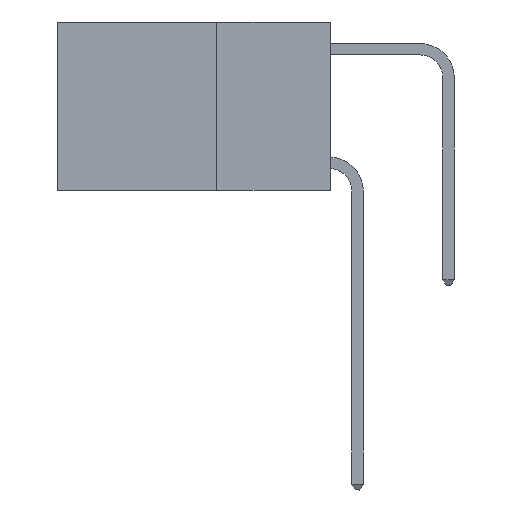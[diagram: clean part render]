
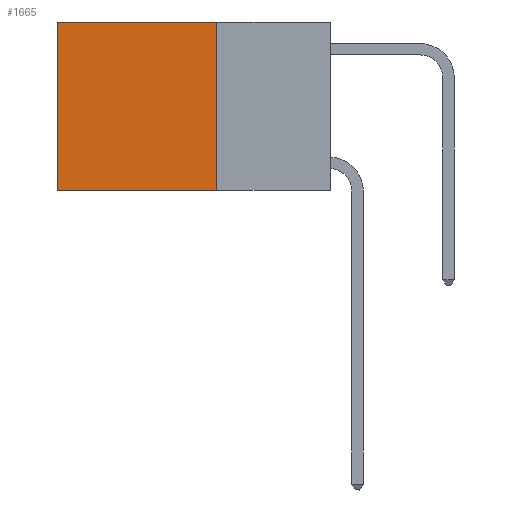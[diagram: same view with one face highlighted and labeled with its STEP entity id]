
A CAD part, left-side view. The second image highlights one B-rep face of the part: STEP entity #1665.
In plain terms, the highlighted planar face has unit normal (-1, 0, 0).
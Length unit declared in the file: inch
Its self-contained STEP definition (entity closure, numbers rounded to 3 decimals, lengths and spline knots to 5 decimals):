
#321 = CARTESIAN_POINT ( 'NONE',  ( 0.2625, 0.25, 0. ) ) ;
#645 = VERTEX_POINT ( 'NONE', #1458 ) ;
#806 = CARTESIAN_POINT ( 'NONE',  ( 0.2625, 0.25, 0. ) ) ;
#1071 = EDGE_CURVE ( 'NONE', #1462, #13157, #5815, .T. ) ;
#1458 = CARTESIAN_POINT ( 'NONE',  ( 0.2625, 0.25, -0.37 ) ) ;
#1462 = VERTEX_POINT ( 'NONE', #11399 ) ;
#1665 = ADVANCED_FACE ( 'NONE', ( #7680 ), #9579, .F. ) ;
#1980 = ORIENTED_EDGE ( 'NONE', *, *, #11956, .F. ) ;
#2825 = VECTOR ( 'NONE', #4287, 39.37008 ) ;
#3129 = ORIENTED_EDGE ( 'NONE', *, *, #9845, .F. ) ;
#3473 = CARTESIAN_POINT ( 'NONE',  ( 0.2625, 0.25, -0.37 ) ) ;
#3650 = AXIS2_PLACEMENT_3D ( 'NONE', #9532, #11773, #5239 ) ;
#3953 = VERTEX_POINT ( 'NONE', #7006 ) ;
#4017 = VECTOR ( 'NONE', #12225, 39.37008 ) ;
#4287 = DIRECTION ( 'NONE',  ( 0., 1., 0. ) ) ;
#4433 = LINE ( 'NONE', #5861, #7014 ) ;
#4465 = CARTESIAN_POINT ( 'NONE',  ( 0.2625, 0.6, 0. ) ) ;
#5239 = DIRECTION ( 'NONE',  ( 0., 0., -1. ) ) ;
#5815 = LINE ( 'NONE', #806, #2825 ) ;
#5861 = CARTESIAN_POINT ( 'NONE',  ( 0.2625, 0.6, 0. ) ) ;
#6144 = LINE ( 'NONE', #321, #14117 ) ;
#7006 = CARTESIAN_POINT ( 'NONE',  ( 0.2625, 0.6, -0.37 ) ) ;
#7014 = VECTOR ( 'NONE', #12363, 39.37008 ) ;
#7680 = FACE_OUTER_BOUND ( 'NONE', #12498, .T. ) ;
#9129 = EDGE_CURVE ( 'NONE', #13157, #3953, #4433, .T. ) ;
#9277 = DIRECTION ( 'NONE',  ( 0., 0., -1. ) ) ;
#9532 = CARTESIAN_POINT ( 'NONE',  ( 0.2625, 0.25, 0. ) ) ;
#9579 = PLANE ( 'NONE',  #3650 ) ;
#9845 = EDGE_CURVE ( 'NONE', #1462, #645, #6144, .T. ) ;
#10166 = LINE ( 'NONE', #3473, #4017 ) ;
#10486 = ORIENTED_EDGE ( 'NONE', *, *, #9129, .T. ) ;
#11399 = CARTESIAN_POINT ( 'NONE',  ( 0.2625, 0.25, 0. ) ) ;
#11773 = DIRECTION ( 'NONE',  ( 1., 0., 0. ) ) ;
#11956 = EDGE_CURVE ( 'NONE', #645, #3953, #10166, .T. ) ;
#12225 = DIRECTION ( 'NONE',  ( 0., 1., 0. ) ) ;
#12363 = DIRECTION ( 'NONE',  ( 0., 0., -1. ) ) ;
#12498 = EDGE_LOOP ( 'NONE', ( #10486, #1980, #3129, #14326 ) ) ;
#13157 = VERTEX_POINT ( 'NONE', #4465 ) ;
#14117 = VECTOR ( 'NONE', #9277, 39.37008 ) ;
#14326 = ORIENTED_EDGE ( 'NONE', *, *, #1071, .T. ) ;
